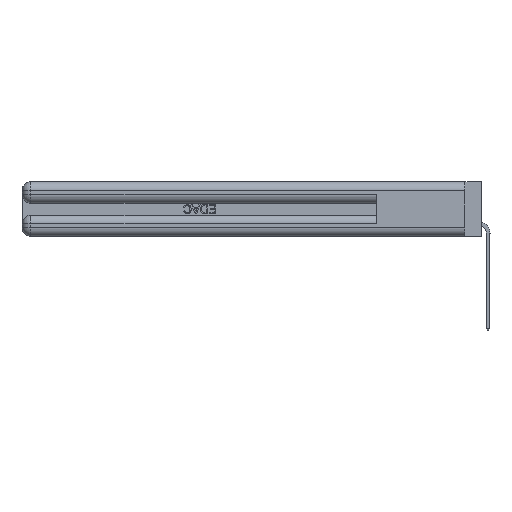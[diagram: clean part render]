
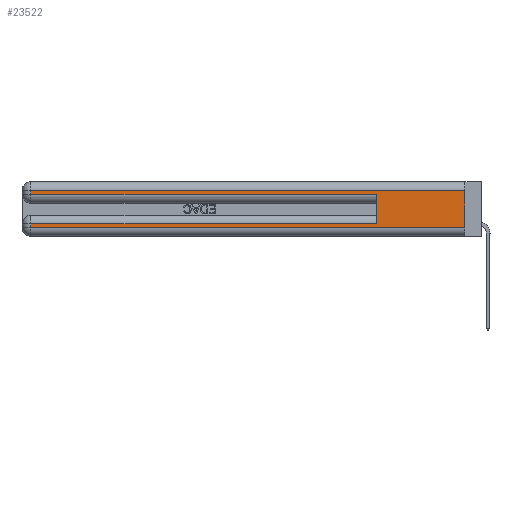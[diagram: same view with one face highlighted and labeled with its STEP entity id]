
A CAD part, left-side view. The second image highlights one B-rep face of the part: STEP entity #23522.
In plain terms, the highlighted planar face has unit normal (-1, 0, 0).
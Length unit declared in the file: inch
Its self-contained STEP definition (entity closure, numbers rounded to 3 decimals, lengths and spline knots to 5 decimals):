
#990 = VECTOR ( 'NONE', #36449, 39.37008 ) ;
#1176 = DIRECTION ( 'NONE',  ( 0., 0., -1. ) ) ;
#1852 = LINE ( 'NONE', #39934, #38128 ) ;
#2526 = CARTESIAN_POINT ( 'NONE',  ( 0., 0., 0.31 ) ) ;
#4009 = CARTESIAN_POINT ( 'NONE',  ( 0., 0., 0.06 ) ) ;
#4128 = VECTOR ( 'NONE', #37253, 39.37008 ) ;
#4169 = LINE ( 'NONE', #19966, #4128 ) ;
#4508 = CARTESIAN_POINT ( 'NONE',  ( 0., 0., 0.085 ) ) ;
#4778 = VERTEX_POINT ( 'NONE', #40580 ) ;
#5961 = CARTESIAN_POINT ( 'NONE',  ( 0., 2.94, 0.285 ) ) ;
#6388 = LINE ( 'NONE', #15507, #990 ) ;
#8913 = ORIENTED_EDGE ( 'NONE', *, *, #16914, .F. ) ;
#9670 = EDGE_CURVE ( 'NONE', #45751, #46210, #33787, .T. ) ;
#10836 = VERTEX_POINT ( 'NONE', #38137 ) ;
#12427 = EDGE_CURVE ( 'NONE', #4778, #10836, #4169, .T. ) ;
#13268 = EDGE_LOOP ( 'NONE', ( #23266, #28357, #17317, #34176, #8913, #39964, #23296, #19122 ) ) ;
#13782 = VECTOR ( 'NONE', #16500, 39.37008 ) ;
#15424 = AXIS2_PLACEMENT_3D ( 'NONE', #48223, #18512, #1176 ) ;
#15507 = CARTESIAN_POINT ( 'NONE',  ( 0., 0., 0.285 ) ) ;
#16393 = VERTEX_POINT ( 'NONE', #5961 ) ;
#16500 = DIRECTION ( 'NONE',  ( 0., -1., 0. ) ) ;
#16861 = CARTESIAN_POINT ( 'NONE',  ( 0., 0.6, 0.085 ) ) ;
#16914 = EDGE_CURVE ( 'NONE', #27813, #30637, #1852, .T. ) ;
#17317 = ORIENTED_EDGE ( 'NONE', *, *, #48387, .T. ) ;
#18512 = DIRECTION ( 'NONE',  ( 1., 0., 0. ) ) ;
#19122 = ORIENTED_EDGE ( 'NONE', *, *, #43097, .T. ) ;
#19966 = CARTESIAN_POINT ( 'NONE',  ( 0., 2.94, 0.37 ) ) ;
#21846 = VECTOR ( 'NONE', #42605, 39.37008 ) ;
#23266 = ORIENTED_EDGE ( 'NONE', *, *, #53867, .F. ) ;
#23296 = ORIENTED_EDGE ( 'NONE', *, *, #12427, .T. ) ;
#23423 = DIRECTION ( 'NONE',  ( 0., 1., 0. ) ) ;
#23522 = ADVANCED_FACE ( 'NONE', ( #35337 ), #52244, .F. ) ;
#25004 = EDGE_CURVE ( 'NONE', #27813, #4778, #39318, .T. ) ;
#26883 = CARTESIAN_POINT ( 'NONE',  ( 0., 0.6, 0.285 ) ) ;
#26952 = CARTESIAN_POINT ( 'NONE',  ( 0., 0., 0.37 ) ) ;
#27813 = VERTEX_POINT ( 'NONE', #16861 ) ;
#27905 = LINE ( 'NONE', #26952, #42355 ) ;
#28357 = ORIENTED_EDGE ( 'NONE', *, *, #9670, .T. ) ;
#28547 = LINE ( 'NONE', #29782, #21846 ) ;
#29782 = CARTESIAN_POINT ( 'NONE',  ( 0., 2.94, 0.37 ) ) ;
#30488 = DIRECTION ( 'NONE',  ( 0., 1., 0. ) ) ;
#30637 = VERTEX_POINT ( 'NONE', #26883 ) ;
#31497 = CARTESIAN_POINT ( 'NONE',  ( 0., 0., 0.31 ) ) ;
#32516 = VECTOR ( 'NONE', #23423, 39.37008 ) ;
#33311 = VERTEX_POINT ( 'NONE', #35538 ) ;
#33787 = LINE ( 'NONE', #31497, #32516 ) ;
#34176 = ORIENTED_EDGE ( 'NONE', *, *, #51408, .T. ) ;
#34798 = CARTESIAN_POINT ( 'NONE',  ( 0., 2.94, 0.31 ) ) ;
#35337 = FACE_OUTER_BOUND ( 'NONE', #13268, .T. ) ;
#35538 = CARTESIAN_POINT ( 'NONE',  ( 0., 0., 0.06 ) ) ;
#36449 = DIRECTION ( 'NONE',  ( 0., -1., 0. ) ) ;
#37253 = DIRECTION ( 'NONE',  ( 0., 0., -1. ) ) ;
#38128 = VECTOR ( 'NONE', #40324, 39.37008 ) ;
#38137 = CARTESIAN_POINT ( 'NONE',  ( 0., 2.94, 0.06 ) ) ;
#39318 = LINE ( 'NONE', #4508, #51052 ) ;
#39934 = CARTESIAN_POINT ( 'NONE',  ( 0., 0.6, 0.145 ) ) ;
#39964 = ORIENTED_EDGE ( 'NONE', *, *, #25004, .T. ) ;
#40324 = DIRECTION ( 'NONE',  ( 0., 0., 1. ) ) ;
#40580 = CARTESIAN_POINT ( 'NONE',  ( 0., 2.94, 0.085 ) ) ;
#42355 = VECTOR ( 'NONE', #47774, 39.37008 ) ;
#42605 = DIRECTION ( 'NONE',  ( 0., 0., -1. ) ) ;
#43097 = EDGE_CURVE ( 'NONE', #10836, #33311, #53937, .T. ) ;
#45751 = VERTEX_POINT ( 'NONE', #2526 ) ;
#46210 = VERTEX_POINT ( 'NONE', #34798 ) ;
#47774 = DIRECTION ( 'NONE',  ( 0., 0., -1. ) ) ;
#48223 = CARTESIAN_POINT ( 'NONE',  ( 0., 0., 0.37 ) ) ;
#48387 = EDGE_CURVE ( 'NONE', #46210, #16393, #28547, .T. ) ;
#51052 = VECTOR ( 'NONE', #30488, 39.37008 ) ;
#51408 = EDGE_CURVE ( 'NONE', #16393, #30637, #6388, .T. ) ;
#52244 = PLANE ( 'NONE',  #15424 ) ;
#53867 = EDGE_CURVE ( 'NONE', #45751, #33311, #27905, .T. ) ;
#53937 = LINE ( 'NONE', #4009, #13782 ) ;
